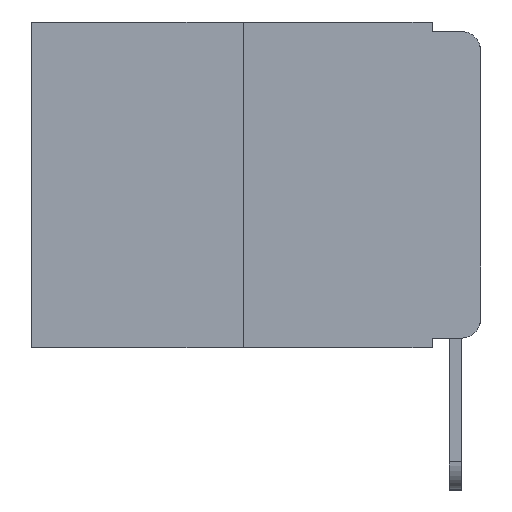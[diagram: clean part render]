
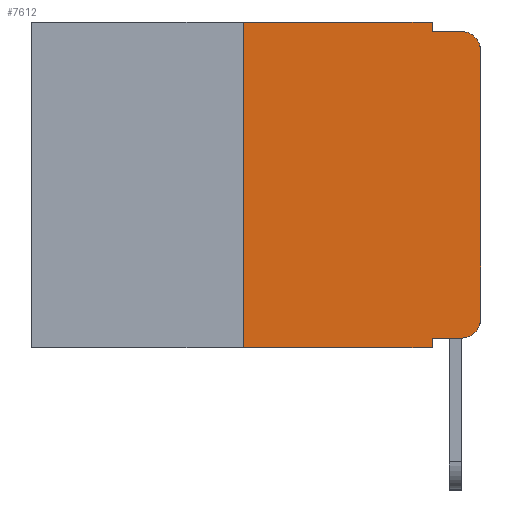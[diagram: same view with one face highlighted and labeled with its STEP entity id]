
A CAD part, left-side view. The second image highlights one B-rep face of the part: STEP entity #7612.
In plain terms, the highlighted planar face has unit normal (-1, 0, 0).
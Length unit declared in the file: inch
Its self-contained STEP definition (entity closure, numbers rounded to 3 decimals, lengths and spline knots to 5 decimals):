
#41 = EDGE_CURVE ( 'NONE', #6126, #1613, #10391, .T. ) ;
#93 = LINE ( 'NONE', #11949, #2888 ) ;
#287 = AXIS2_PLACEMENT_3D ( 'NONE', #12205, #2963, #10267 ) ;
#449 = VERTEX_POINT ( 'NONE', #12580 ) ;
#585 = AXIS2_PLACEMENT_3D ( 'NONE', #2032, #9411, #3116 ) ;
#705 = FACE_OUTER_BOUND ( 'NONE', #10768, .T. ) ;
#738 = EDGE_CURVE ( 'NONE', #1182, #861, #8831, .T. ) ;
#761 = CARTESIAN_POINT ( 'NONE',  ( 0., 0., 0. ) ) ;
#861 = VERTEX_POINT ( 'NONE', #6868 ) ;
#980 = CARTESIAN_POINT ( 'NONE',  ( 0., 0.473, -0.343 ) ) ;
#1182 = VERTEX_POINT ( 'NONE', #5480 ) ;
#1613 = VERTEX_POINT ( 'NONE', #5330 ) ;
#1853 = DIRECTION ( 'NONE',  ( 0., 0., -1. ) ) ;
#1889 = AXIS2_PLACEMENT_3D ( 'NONE', #3057, #11857, #11774 ) ;
#2023 = EDGE_CURVE ( 'NONE', #861, #12589, #6365, .T. ) ;
#2032 = CARTESIAN_POINT ( 'NONE',  ( 0., 0.02, -0.03 ) ) ;
#2119 = EDGE_CURVE ( 'NONE', #449, #13527, #8141, .T. ) ;
#2134 = EDGE_CURVE ( 'NONE', #449, #1613, #13147, .T. ) ;
#2186 = VECTOR ( 'NONE', #11532, 39.37008 ) ;
#2307 = VECTOR ( 'NONE', #12190, 39.37008 ) ;
#2515 = ORIENTED_EDGE ( 'NONE', *, *, #738, .T. ) ;
#2817 = EDGE_CURVE ( 'NONE', #12589, #10307, #4675, .T. ) ;
#2868 = CARTESIAN_POINT ( 'NONE',  ( 0., 0.473, 0. ) ) ;
#2888 = VECTOR ( 'NONE', #6901, 39.37008 ) ;
#2963 = DIRECTION ( 'NONE',  ( 1., 0., 0. ) ) ;
#3010 = ORIENTED_EDGE ( 'NONE', *, *, #2119, .F. ) ;
#3057 = CARTESIAN_POINT ( 'NONE',  ( 0., 0.02, -0.313 ) ) ;
#3116 = DIRECTION ( 'NONE',  ( 0., 0., -1. ) ) ;
#3335 = CARTESIAN_POINT ( 'NONE',  ( 0., 0.051, 0. ) ) ;
#3677 = ORIENTED_EDGE ( 'NONE', *, *, #8906, .T. ) ;
#3845 = ORIENTED_EDGE ( 'NONE', *, *, #41, .F. ) ;
#3987 = VERTEX_POINT ( 'NONE', #4471 ) ;
#4471 = CARTESIAN_POINT ( 'NONE',  ( 0., 0.051, -0.01 ) ) ;
#4675 = CIRCLE ( 'NONE', #585, 0.02 ) ;
#4896 = VECTOR ( 'NONE', #1853, 39.37008 ) ;
#5029 = VECTOR ( 'NONE', #6398, 39.37008 ) ;
#5260 = VECTOR ( 'NONE', #9425, 39.37008 ) ;
#5330 = CARTESIAN_POINT ( 'NONE',  ( 0., 0.051, -0.343 ) ) ;
#5480 = CARTESIAN_POINT ( 'NONE',  ( 0., 0.02, -0.333 ) ) ;
#5590 = LINE ( 'NONE', #8384, #5260 ) ;
#5684 = CARTESIAN_POINT ( 'NONE',  ( 0., 0.051, 0. ) ) ;
#6119 = CARTESIAN_POINT ( 'NONE',  ( 0., 0.051, -0.01 ) ) ;
#6126 = VERTEX_POINT ( 'NONE', #7183 ) ;
#6318 = CARTESIAN_POINT ( 'NONE',  ( 0., 0.25, 0. ) ) ;
#6365 = LINE ( 'NONE', #761, #9111 ) ;
#6398 = DIRECTION ( 'NONE',  ( 0., 0., 1. ) ) ;
#6441 = CARTESIAN_POINT ( 'NONE',  ( 0., 0.25, 0. ) ) ;
#6868 = CARTESIAN_POINT ( 'NONE',  ( 0., 0., -0.313 ) ) ;
#6901 = DIRECTION ( 'NONE',  ( 0., 0., -1. ) ) ;
#7037 = VECTOR ( 'NONE', #7075, 39.37008 ) ;
#7075 = DIRECTION ( 'NONE',  ( 0., -1., 0. ) ) ;
#7125 = ORIENTED_EDGE ( 'NONE', *, *, #2817, .T. ) ;
#7183 = CARTESIAN_POINT ( 'NONE',  ( 0., 0.051, -0.333 ) ) ;
#7369 = LINE ( 'NONE', #2868, #7037 ) ;
#7451 = EDGE_CURVE ( 'NONE', #8566, #3987, #93, .T. ) ;
#7612 = ADVANCED_FACE ( 'NONE', ( #705 ), #9273, .F. ) ;
#7810 = ORIENTED_EDGE ( 'NONE', *, *, #13428, .F. ) ;
#7838 = CARTESIAN_POINT ( 'NONE',  ( 0., 0., -0.03 ) ) ;
#8141 = LINE ( 'NONE', #6441, #5029 ) ;
#8384 = CARTESIAN_POINT ( 'NONE',  ( 0., 0.051, -0.333 ) ) ;
#8566 = VERTEX_POINT ( 'NONE', #5684 ) ;
#8831 = CIRCLE ( 'NONE', #1889, 0.02 ) ;
#8906 = EDGE_CURVE ( 'NONE', #6126, #1182, #5590, .T. ) ;
#8942 = ORIENTED_EDGE ( 'NONE', *, *, #9444, .F. ) ;
#9111 = VECTOR ( 'NONE', #12305, 39.37008 ) ;
#9273 = PLANE ( 'NONE',  #287 ) ;
#9411 = DIRECTION ( 'NONE',  ( -1., 0., 0. ) ) ;
#9425 = DIRECTION ( 'NONE',  ( 0., -1., 0. ) ) ;
#9444 = EDGE_CURVE ( 'NONE', #13527, #8566, #7369, .T. ) ;
#9471 = ORIENTED_EDGE ( 'NONE', *, *, #2023, .T. ) ;
#9598 = ORIENTED_EDGE ( 'NONE', *, *, #7451, .F. ) ;
#10267 = DIRECTION ( 'NONE',  ( 0., 0., -1. ) ) ;
#10307 = VERTEX_POINT ( 'NONE', #12183 ) ;
#10391 = LINE ( 'NONE', #3335, #4896 ) ;
#10619 = LINE ( 'NONE', #6119, #2307 ) ;
#10768 = EDGE_LOOP ( 'NONE', ( #9471, #7125, #7810, #9598, #8942, #3010, #12346, #3845, #3677, #2515 ) ) ;
#11532 = DIRECTION ( 'NONE',  ( 0., -1., 0. ) ) ;
#11774 = DIRECTION ( 'NONE',  ( 0., 0., -1. ) ) ;
#11857 = DIRECTION ( 'NONE',  ( -1., 0., 0. ) ) ;
#11949 = CARTESIAN_POINT ( 'NONE',  ( 0., 0.051, 0. ) ) ;
#12183 = CARTESIAN_POINT ( 'NONE',  ( 0., 0.02, -0.01 ) ) ;
#12190 = DIRECTION ( 'NONE',  ( 0., -1., 0. ) ) ;
#12205 = CARTESIAN_POINT ( 'NONE',  ( 0., 0.473, 0. ) ) ;
#12305 = DIRECTION ( 'NONE',  ( 0., 0., 1. ) ) ;
#12346 = ORIENTED_EDGE ( 'NONE', *, *, #2134, .T. ) ;
#12580 = CARTESIAN_POINT ( 'NONE',  ( 0., 0.25, -0.343 ) ) ;
#12589 = VERTEX_POINT ( 'NONE', #7838 ) ;
#13147 = LINE ( 'NONE', #980, #2186 ) ;
#13428 = EDGE_CURVE ( 'NONE', #3987, #10307, #10619, .T. ) ;
#13527 = VERTEX_POINT ( 'NONE', #6318 ) ;
